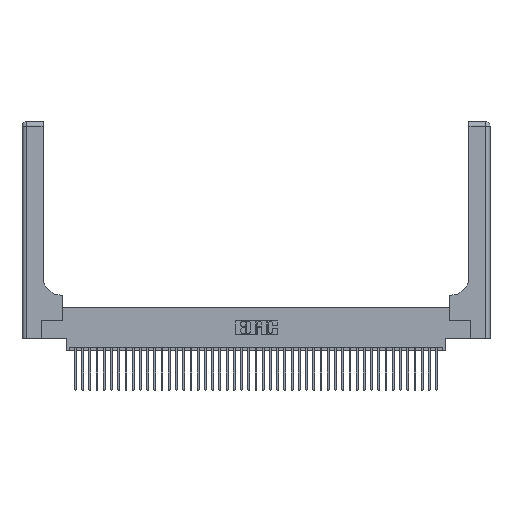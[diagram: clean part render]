
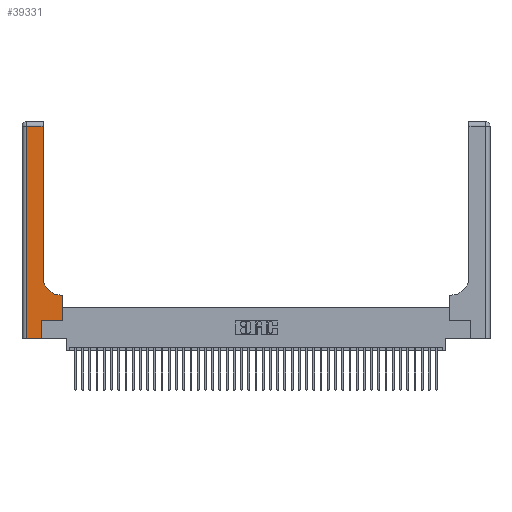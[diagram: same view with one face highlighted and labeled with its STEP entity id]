
A CAD part, top view. The second image highlights one B-rep face of the part: STEP entity #39331.
In plain terms, the highlighted planar face has unit normal (0, 0, 1).
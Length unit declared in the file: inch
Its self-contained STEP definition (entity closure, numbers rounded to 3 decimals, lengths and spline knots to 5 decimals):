
#1016 = DIRECTION ( 'NONE',  ( -1., 0., 0. ) ) ;
#1955 = DIRECTION ( 'NONE',  ( 0., 0., -1. ) ) ;
#2115 = VECTOR ( 'NONE', #34277, 39.37008 ) ;
#2974 = CARTESIAN_POINT ( 'NONE',  ( 0., 0., 0.37 ) ) ;
#3048 = VERTEX_POINT ( 'NONE', #41926 ) ;
#3920 = AXIS2_PLACEMENT_3D ( 'NONE', #38814, #18390, #14828 ) ;
#4440 = ORIENTED_EDGE ( 'NONE', *, *, #5622, .T. ) ;
#4791 = EDGE_CURVE ( 'NONE', #16879, #22038, #8322, .T. ) ;
#5622 = EDGE_CURVE ( 'NONE', #17450, #3048, #36042, .T. ) ;
#6575 = DIRECTION ( 'NONE',  ( 0., 1., 0. ) ) ;
#8131 = FACE_OUTER_BOUND ( 'NONE', #28605, .T. ) ;
#8322 = LINE ( 'NONE', #41344, #34467 ) ;
#8563 = VECTOR ( 'NONE', #14511, 39.37008 ) ;
#8662 = PLANE ( 'NONE',  #33257 ) ;
#8819 = LINE ( 'NONE', #8823, #24790 ) ;
#8823 = CARTESIAN_POINT ( 'NONE',  ( 0., 2.94, 0.37 ) ) ;
#9512 = VERTEX_POINT ( 'NONE', #9920 ) ;
#9591 = CARTESIAN_POINT ( 'NONE',  ( 0.5585, 0.25, 0.37 ) ) ;
#9714 = EDGE_CURVE ( 'NONE', #22038, #40304, #8819, .T. ) ;
#9920 = CARTESIAN_POINT ( 'NONE',  ( 0.269, 0., 0.37 ) ) ;
#9927 = CARTESIAN_POINT ( 'NONE',  ( 0.5415, 0.6, 0.37 ) ) ;
#10446 = VECTOR ( 'NONE', #1016, 39.37008 ) ;
#11414 = VERTEX_POINT ( 'NONE', #9927 ) ;
#14511 = DIRECTION ( 'NONE',  ( 0., -1., 0. ) ) ;
#14828 = DIRECTION ( 'NONE',  ( 1., 0., 0. ) ) ;
#15503 = VECTOR ( 'NONE', #41651, 39.37008 ) ;
#16047 = LINE ( 'NONE', #24803, #15503 ) ;
#16879 = VERTEX_POINT ( 'NONE', #39889 ) ;
#17267 = ORIENTED_EDGE ( 'NONE', *, *, #28746, .T. ) ;
#17450 = VERTEX_POINT ( 'NONE', #43202 ) ;
#17828 = DIRECTION ( 'NONE',  ( 0., 1., 0. ) ) ;
#18390 = DIRECTION ( 'NONE',  ( 0., 0., -1. ) ) ;
#19541 = LINE ( 'NONE', #31877, #10446 ) ;
#21363 = LINE ( 'NONE', #37421, #2115 ) ;
#21890 = CARTESIAN_POINT ( 'NONE',  ( 0.06, 2.94, 0.37 ) ) ;
#22038 = VERTEX_POINT ( 'NONE', #43411 ) ;
#22618 = ORIENTED_EDGE ( 'NONE', *, *, #39365, .T. ) ;
#22720 = ORIENTED_EDGE ( 'NONE', *, *, #41755, .T. ) ;
#22977 = CARTESIAN_POINT ( 'NONE',  ( 0., 3., 0.37 ) ) ;
#23356 = VERTEX_POINT ( 'NONE', #34644 ) ;
#24007 = CIRCLE ( 'NONE', #3920, 0.25 ) ;
#24637 = LINE ( 'NONE', #2974, #33230 ) ;
#24653 = ORIENTED_EDGE ( 'NONE', *, *, #9714, .T. ) ;
#24790 = VECTOR ( 'NONE', #42979, 39.37008 ) ;
#24803 = CARTESIAN_POINT ( 'NONE',  ( 0.269, 0., 0.37 ) ) ;
#25627 = ORIENTED_EDGE ( 'NONE', *, *, #40698, .T. ) ;
#28605 = EDGE_LOOP ( 'NONE', ( #35358, #24653, #17267, #22618, #25627, #22720, #4440, #33916, #32867 ) ) ;
#28746 = EDGE_CURVE ( 'NONE', #40304, #23356, #30439, .T. ) ;
#29241 = DIRECTION ( 'NONE',  ( -1., 0., 0. ) ) ;
#30439 = LINE ( 'NONE', #38512, #8563 ) ;
#31877 = CARTESIAN_POINT ( 'NONE',  ( 0.2915, 0.6, 0.37 ) ) ;
#32748 = CARTESIAN_POINT ( 'NONE',  ( 0.269, 0.25, 0.37 ) ) ;
#32867 = ORIENTED_EDGE ( 'NONE', *, *, #35057, .T. ) ;
#33230 = VECTOR ( 'NONE', #44140, 39.37008 ) ;
#33257 = AXIS2_PLACEMENT_3D ( 'NONE', #22977, #1955, #29241 ) ;
#33916 = ORIENTED_EDGE ( 'NONE', *, *, #37935, .T. ) ;
#34277 = DIRECTION ( 'NONE',  ( 1., 0., 0. ) ) ;
#34467 = VECTOR ( 'NONE', #17828, 39.37008 ) ;
#34644 = CARTESIAN_POINT ( 'NONE',  ( 0.06, 0., 0.37 ) ) ;
#35057 = EDGE_CURVE ( 'NONE', #11414, #16879, #24007, .T. ) ;
#35358 = ORIENTED_EDGE ( 'NONE', *, *, #4791, .T. ) ;
#36042 = LINE ( 'NONE', #9591, #41861 ) ;
#37421 = CARTESIAN_POINT ( 'NONE',  ( 0.269, 0.25, 0.37 ) ) ;
#37935 = EDGE_CURVE ( 'NONE', #3048, #11414, #19541, .T. ) ;
#38512 = CARTESIAN_POINT ( 'NONE',  ( 0.06, 3., 0.37 ) ) ;
#38624 = VERTEX_POINT ( 'NONE', #32748 ) ;
#38814 = CARTESIAN_POINT ( 'NONE',  ( 0.5415, 0.85, 0.37 ) ) ;
#39331 = ADVANCED_FACE ( 'NONE', ( #8131 ), #8662, .F. ) ;
#39365 = EDGE_CURVE ( 'NONE', #23356, #9512, #24637, .T. ) ;
#39889 = CARTESIAN_POINT ( 'NONE',  ( 0.2915, 0.85, 0.37 ) ) ;
#40304 = VERTEX_POINT ( 'NONE', #21890 ) ;
#40698 = EDGE_CURVE ( 'NONE', #9512, #38624, #16047, .T. ) ;
#41344 = CARTESIAN_POINT ( 'NONE',  ( 0.2915, 3., 0.37 ) ) ;
#41651 = DIRECTION ( 'NONE',  ( 0., 1., 0. ) ) ;
#41755 = EDGE_CURVE ( 'NONE', #38624, #17450, #21363, .T. ) ;
#41861 = VECTOR ( 'NONE', #6575, 39.37008 ) ;
#41926 = CARTESIAN_POINT ( 'NONE',  ( 0.5585, 0.6, 0.37 ) ) ;
#42979 = DIRECTION ( 'NONE',  ( -1., 0., 0. ) ) ;
#43202 = CARTESIAN_POINT ( 'NONE',  ( 0.5585, 0.25, 0.37 ) ) ;
#43411 = CARTESIAN_POINT ( 'NONE',  ( 0.2915, 2.94, 0.37 ) ) ;
#44140 = DIRECTION ( 'NONE',  ( 1., 0., 0. ) ) ;
